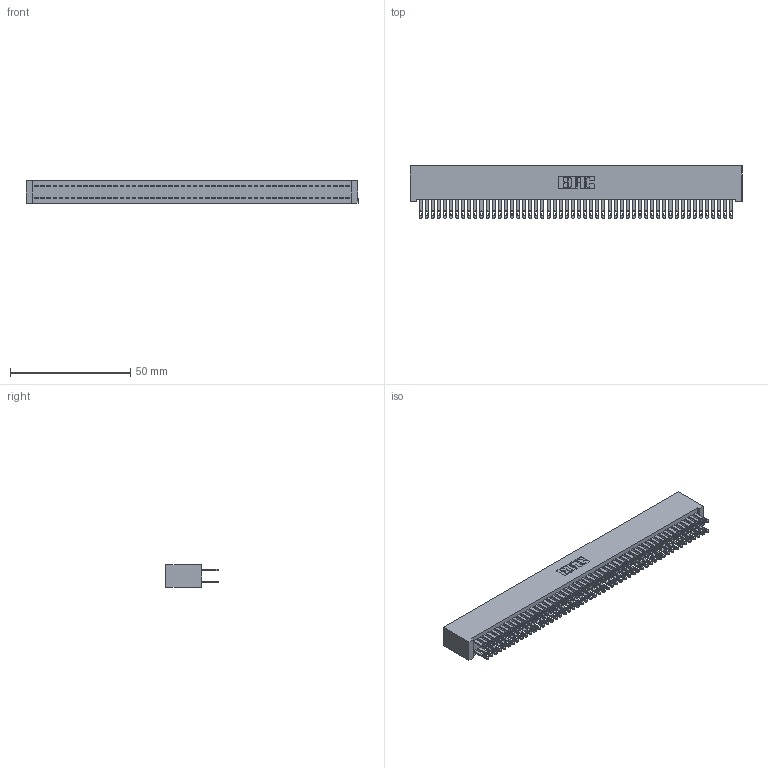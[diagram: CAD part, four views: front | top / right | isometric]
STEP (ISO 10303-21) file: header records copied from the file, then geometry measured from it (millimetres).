
FILE_DESCRIPTION (( 'STEP AP203' ), '1' );
FILE_NAME ('892-104-500-201.STEP', '2020-09-21T21:29:51', ( '' ), ( '' ), 'SwSTEP 2.0', 'SolidWorks 2020', '' );
FILE_SCHEMA (( 'CONFIG_CONTROL_DESIGN' ));
Length unit declared in the file: inch
Products named in the file (3): 345-292-001_345-293-100; 892-104-500-201; 842 Part_Lugless
Assembly tree (105 placements, depth 2):
  892-104-500-201
    842 Part_Lugless
    345-292-001_345-293-100  x104
Bounding box: 138.33 x 21.85 x 9.4 mm (x, y, z)
Volume: 13233.4 mm3; surface area: 23229.1 mm2
Topology: 105 solids, 105 shells, 5094 faces, 15563 edges, 10374 vertices
Faces by surface type: plane 3182, cylinder 1912
Entity records: 31681 total; most frequent: CARTESIAN_POINT 5234, ORIENTED_EDGE 5170, DIRECTION 4449, EDGE_CURVE 2585, LINE 2461, VECTOR 2461, VERTEX_POINT 1722, AXIS2_PLACEMENT_3D 994
